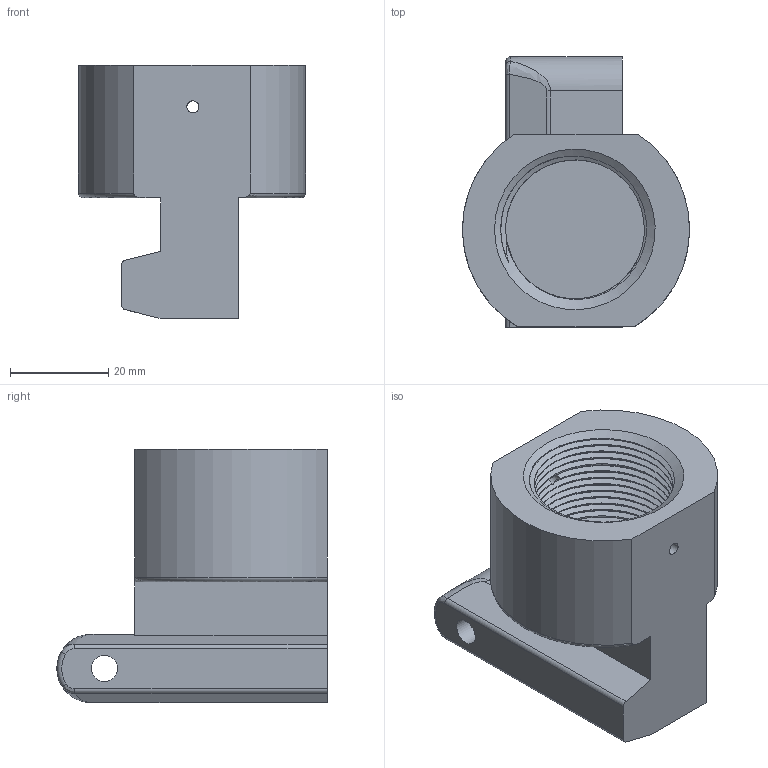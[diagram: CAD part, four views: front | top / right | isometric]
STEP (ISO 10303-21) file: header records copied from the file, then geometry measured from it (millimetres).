
FILE_DESCRIPTION(/* description */ (''),/* implementation_level */ '2;1');
FILE_NAME(/* name */ 'WTF FOLDING STOCK ADAPTER.stp',/* time_stamp */ '2020-05-06T19:15:04+03:00',/* author */ (''),/* organization */ (''),/* preprocessor_version */ 'ST-DEVELOPER v15.2',/* originating_system */ 'Autodesk Translator Framework v2.0.0.5431',/* authorisation */ '');
FILE_SCHEMA (('AUTOMOTIVE_DESIGN { 1 0 10303 214 3 1 1 }'));
Length unit declared in the file: centimetre
Products named in the file (1): FOLDING STOCK ADAPTOR AR15-M4
Bounding box: 46.16 x 54.96 x 51.45 mm (x, y, z)
Volume: 50739.3 mm3; surface area: 14738.2 mm2
Topology: 1 solids, 1 shells, 62 faces, 241 edges, 180 vertices
Faces by surface type: bspline 24, plane 20, cylinder 14, torus 3, cone 1
Full cylindrical faces by diameter (mm): 2.475 x2, 5.346 x1
Entity records: 16947 total; most frequent: CARTESIAN_POINT 15289, ORIENTED_EDGE 468, EDGE_CURVE 234, DIRECTION 185, VERTEX_POINT 177, B_SPLINE_CURVE_WITH_KNOTS 142, AXIS2_PLACEMENT_3D 74, EDGE_LOOP 71
